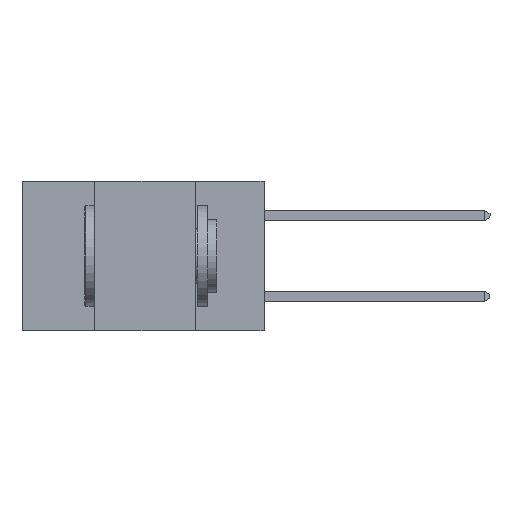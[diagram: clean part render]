
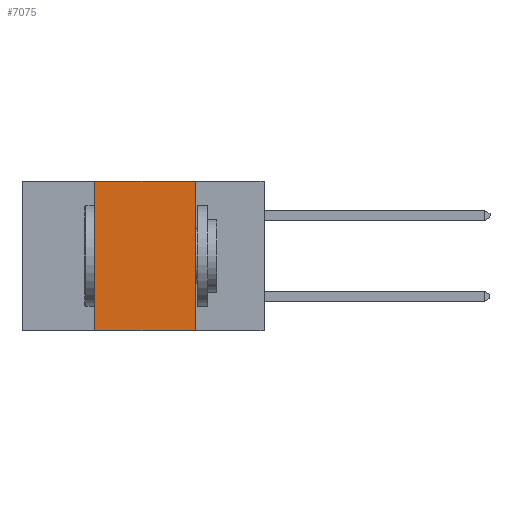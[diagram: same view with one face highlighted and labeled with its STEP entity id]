
A CAD part, left-side view. The second image highlights one B-rep face of the part: STEP entity #7075.
In plain terms, the highlighted planar face has unit normal (-1, 0, 0).
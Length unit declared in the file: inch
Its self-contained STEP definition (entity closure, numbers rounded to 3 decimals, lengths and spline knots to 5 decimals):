
#255 = CARTESIAN_POINT ( 'NONE',  ( 0., 0.6, 0. ) ) ;
#307 = AXIS2_PLACEMENT_3D ( 'NONE', #7171, #25868, #13419 ) ;
#975 = VERTEX_POINT ( 'NONE', #1306 ) ;
#1306 = CARTESIAN_POINT ( 'NONE',  ( 0., 0.17, 0. ) ) ;
#2584 = LINE ( 'NONE', #11675, #13617 ) ;
#4748 = VERTEX_POINT ( 'NONE', #7330 ) ;
#6346 = EDGE_CURVE ( 'NONE', #18782, #19723, #21851, .T. ) ;
#6847 = DIRECTION ( 'NONE',  ( 0., -1., 0. ) ) ;
#7075 = ADVANCED_FACE ( 'NONE', ( #26020 ), #9248, .F. ) ;
#7171 = CARTESIAN_POINT ( 'NONE',  ( 0., 0.6, 0. ) ) ;
#7330 = CARTESIAN_POINT ( 'NONE',  ( 0., 0.42, 0. ) ) ;
#7974 = DIRECTION ( 'NONE',  ( 0., 0., -1. ) ) ;
#9248 = PLANE ( 'NONE',  #307 ) ;
#10205 = ORIENTED_EDGE ( 'NONE', *, *, #11696, .F. ) ;
#11022 = LINE ( 'NONE', #22528, #26896 ) ;
#11120 = CARTESIAN_POINT ( 'NONE',  ( 0., 0.6, -0.37 ) ) ;
#11587 = DIRECTION ( 'NONE',  ( 0., 0., 1. ) ) ;
#11675 = CARTESIAN_POINT ( 'NONE',  ( 0., 0.42, 0. ) ) ;
#11696 = EDGE_CURVE ( 'NONE', #975, #19723, #11022, .T. ) ;
#12254 = EDGE_CURVE ( 'NONE', #18782, #4748, #2584, .T. ) ;
#12694 = ORIENTED_EDGE ( 'NONE', *, *, #25160, .F. ) ;
#13419 = DIRECTION ( 'NONE',  ( 0., 0., -1. ) ) ;
#13617 = VECTOR ( 'NONE', #11587, 39.37008 ) ;
#14712 = VECTOR ( 'NONE', #14840, 39.37008 ) ;
#14795 = ORIENTED_EDGE ( 'NONE', *, *, #12254, .F. ) ;
#14840 = DIRECTION ( 'NONE',  ( 0., -1., 0. ) ) ;
#16200 = EDGE_LOOP ( 'NONE', ( #10205, #12694, #14795, #20746 ) ) ;
#16255 = VECTOR ( 'NONE', #6847, 39.37008 ) ;
#18782 = VERTEX_POINT ( 'NONE', #19871 ) ;
#19630 = LINE ( 'NONE', #255, #14712 ) ;
#19723 = VERTEX_POINT ( 'NONE', #24746 ) ;
#19871 = CARTESIAN_POINT ( 'NONE',  ( 0., 0.42, -0.37 ) ) ;
#20746 = ORIENTED_EDGE ( 'NONE', *, *, #6346, .T. ) ;
#21851 = LINE ( 'NONE', #11120, #16255 ) ;
#22528 = CARTESIAN_POINT ( 'NONE',  ( 0., 0.17, 0. ) ) ;
#24746 = CARTESIAN_POINT ( 'NONE',  ( 0., 0.17, -0.37 ) ) ;
#25160 = EDGE_CURVE ( 'NONE', #4748, #975, #19630, .T. ) ;
#25868 = DIRECTION ( 'NONE',  ( 1., 0., 0. ) ) ;
#26020 = FACE_OUTER_BOUND ( 'NONE', #16200, .T. ) ;
#26896 = VECTOR ( 'NONE', #7974, 39.37008 ) ;
